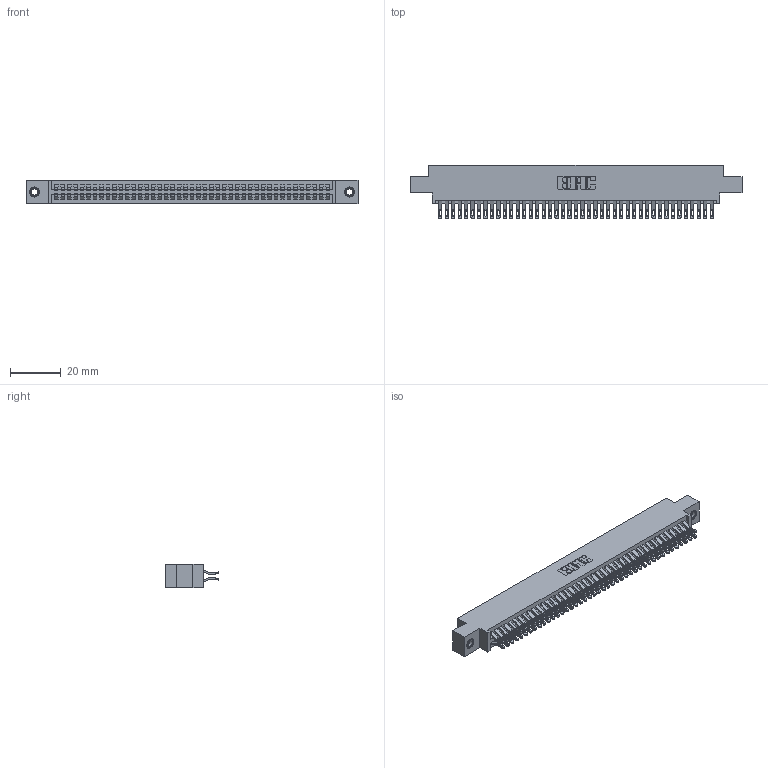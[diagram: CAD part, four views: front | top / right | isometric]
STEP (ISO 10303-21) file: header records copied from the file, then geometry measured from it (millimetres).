
FILE_DESCRIPTION (( 'STEP AP203' ), '1' );
FILE_NAME ('345-086-555-807.STEP', '2019-11-01T08:42:44', ( '' ), ( '' ), 'SwSTEP 2.0', 'SolidWorks 2016', '' );
FILE_SCHEMA (( 'CONFIG_CONTROL_DESIGN' ));
Length unit declared in the file: inch
Products named in the file (4): 345-292-001_555 Tail; 345 Part_0.170 Offset - 0.156 Dia-TI; 345-086-555-807; 345-250-001_345-250-005-103
Assembly tree (89 placements, depth 2):
  345-086-555-807
    345 Part_0.170 Offset - 0.156 Dia-TI
    345-292-001_555 Tail  x86
    345-250-001_345-250-005-103  x2
Bounding box: 130.43 x 21.13 x 9.4 mm (x, y, z)
Volume: 12801.8 mm3; surface area: 19981.6 mm2
Topology: 89 solids, 89 shells, 5006 faces, 15711 edges, 10466 vertices
Faces by surface type: plane 2782, cylinder 2208, cone 12, torus 4
Entity records: 35248 total; most frequent: CARTESIAN_POINT 5925, ORIENTED_EDGE 5822, DIRECTION 5217, EDGE_CURVE 2911, LINE 2567, VECTOR 2567, VERTEX_POINT 1936, AXIS2_PLACEMENT_3D 1325
